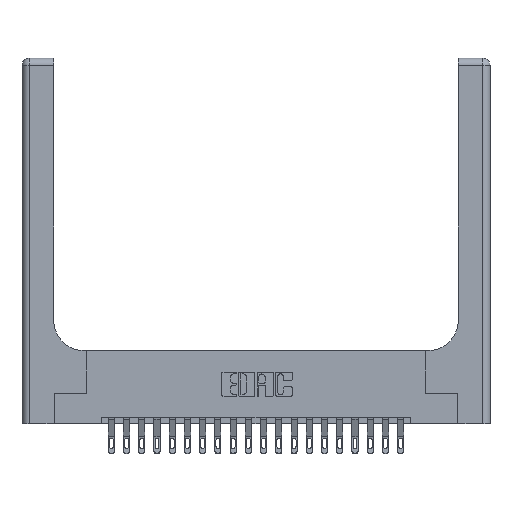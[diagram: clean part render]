
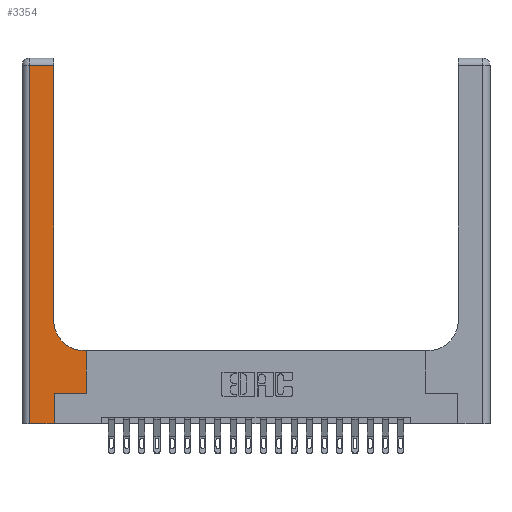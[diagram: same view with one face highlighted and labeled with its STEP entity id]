
A CAD part, top view. The second image highlights one B-rep face of the part: STEP entity #3354.
In plain terms, the highlighted planar face has unit normal (0, 0, 1).
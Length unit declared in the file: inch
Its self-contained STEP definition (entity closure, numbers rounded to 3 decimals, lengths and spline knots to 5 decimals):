
#158 = DIRECTION ( 'NONE',  ( 0., 1., 0. ) ) ;
#617 = DIRECTION ( 'NONE',  ( 0., 1., 0. ) ) ;
#770 = VERTEX_POINT ( 'NONE', #4669 ) ;
#783 = VECTOR ( 'NONE', #617, 39.37008 ) ;
#978 = ORIENTED_EDGE ( 'NONE', *, *, #3199, .T. ) ;
#1184 = CARTESIAN_POINT ( 'NONE',  ( 0.265, 0.25, 0.37 ) ) ;
#1213 = EDGE_CURVE ( 'NONE', #14390, #5880, #8174, .T. ) ;
#1715 = DIRECTION ( 'NONE',  ( 0., 1., 0. ) ) ;
#1854 = VERTEX_POINT ( 'NONE', #5605 ) ;
#2528 = EDGE_CURVE ( 'NONE', #5880, #2581, #20849, .T. ) ;
#2580 = CARTESIAN_POINT ( 'NONE',  ( 0., 0., 0.37 ) ) ;
#2581 = VERTEX_POINT ( 'NONE', #12639 ) ;
#2617 = VECTOR ( 'NONE', #18148, 39.37008 ) ;
#3199 = EDGE_CURVE ( 'NONE', #2581, #13052, #21910, .T. ) ;
#3354 = ADVANCED_FACE ( 'NONE', ( #7127 ), #10811, .F. ) ;
#3676 = VECTOR ( 'NONE', #3851, 39.37008 ) ;
#3730 = LINE ( 'NONE', #15426, #5581 ) ;
#3851 = DIRECTION ( 'NONE',  ( -1., 0., 0. ) ) ;
#4039 = ORIENTED_EDGE ( 'NONE', *, *, #1213, .T. ) ;
#4100 = VECTOR ( 'NONE', #14975, 39.37008 ) ;
#4532 = CARTESIAN_POINT ( 'NONE',  ( 0.51, 0.85, 0.37 ) ) ;
#4669 = CARTESIAN_POINT ( 'NONE',  ( 0.06, 2.94, 0.37 ) ) ;
#5200 = CARTESIAN_POINT ( 'NONE',  ( 0.26, 2.94, 0.37 ) ) ;
#5533 = CARTESIAN_POINT ( 'NONE',  ( 0., 2.94, 0.37 ) ) ;
#5581 = VECTOR ( 'NONE', #158, 39.37008 ) ;
#5605 = CARTESIAN_POINT ( 'NONE',  ( 0.265, 0., 0.37 ) ) ;
#5880 = VERTEX_POINT ( 'NONE', #6760 ) ;
#6688 = VERTEX_POINT ( 'NONE', #11635 ) ;
#6692 = AXIS2_PLACEMENT_3D ( 'NONE', #20903, #9017, #18908 ) ;
#6760 = CARTESIAN_POINT ( 'NONE',  ( 0.528, 0.25, 0.37 ) ) ;
#7127 = FACE_OUTER_BOUND ( 'NONE', #17391, .T. ) ;
#7720 = ORIENTED_EDGE ( 'NONE', *, *, #15344, .T. ) ;
#8174 = LINE ( 'NONE', #18402, #4100 ) ;
#8214 = VERTEX_POINT ( 'NONE', #11285 ) ;
#8620 = VECTOR ( 'NONE', #1715, 39.37008 ) ;
#9017 = DIRECTION ( 'NONE',  ( 0., 0., -1. ) ) ;
#10811 = PLANE ( 'NONE',  #6692 ) ;
#11133 = EDGE_CURVE ( 'NONE', #13052, #8214, #12882, .T. ) ;
#11285 = CARTESIAN_POINT ( 'NONE',  ( 0.26, 0.85, 0.37 ) ) ;
#11506 = CARTESIAN_POINT ( 'NONE',  ( 0.06, 3., 0.37 ) ) ;
#11635 = CARTESIAN_POINT ( 'NONE',  ( 0.06, 0., 0.37 ) ) ;
#11668 = ORIENTED_EDGE ( 'NONE', *, *, #20123, .T. ) ;
#11741 = LINE ( 'NONE', #16849, #8620 ) ;
#12639 = CARTESIAN_POINT ( 'NONE',  ( 0.528, 0.6, 0.37 ) ) ;
#12882 = CIRCLE ( 'NONE', #21733, 0.25 ) ;
#13052 = VERTEX_POINT ( 'NONE', #17190 ) ;
#13332 = ORIENTED_EDGE ( 'NONE', *, *, #13806, .T. ) ;
#13486 = CARTESIAN_POINT ( 'NONE',  ( 0.26, 0.6, 0.37 ) ) ;
#13806 = EDGE_CURVE ( 'NONE', #1854, #14390, #11741, .T. ) ;
#13875 = LINE ( 'NONE', #5533, #3676 ) ;
#14360 = ORIENTED_EDGE ( 'NONE', *, *, #15170, .T. ) ;
#14390 = VERTEX_POINT ( 'NONE', #1184 ) ;
#14546 = EDGE_CURVE ( 'NONE', #21934, #770, #13875, .T. ) ;
#14562 = DIRECTION ( 'NONE',  ( 0., 0., -1. ) ) ;
#14975 = DIRECTION ( 'NONE',  ( 1., 0., 0. ) ) ;
#15170 = EDGE_CURVE ( 'NONE', #6688, #1854, #19482, .T. ) ;
#15344 = EDGE_CURVE ( 'NONE', #770, #6688, #18474, .T. ) ;
#15426 = CARTESIAN_POINT ( 'NONE',  ( 0.26, 3., 0.37 ) ) ;
#15474 = ORIENTED_EDGE ( 'NONE', *, *, #14546, .T. ) ;
#15646 = CARTESIAN_POINT ( 'NONE',  ( 0.528, 0.25, 0.37 ) ) ;
#16166 = DIRECTION ( 'NONE',  ( 1., 0., 0. ) ) ;
#16849 = CARTESIAN_POINT ( 'NONE',  ( 0.265, 0., 0.37 ) ) ;
#16992 = ORIENTED_EDGE ( 'NONE', *, *, #11133, .T. ) ;
#17190 = CARTESIAN_POINT ( 'NONE',  ( 0.51, 0.6, 0.37 ) ) ;
#17391 = EDGE_LOOP ( 'NONE', ( #11668, #15474, #7720, #14360, #13332, #4039, #17827, #978, #16992 ) ) ;
#17827 = ORIENTED_EDGE ( 'NONE', *, *, #2528, .T. ) ;
#18148 = DIRECTION ( 'NONE',  ( 0., -1., 0. ) ) ;
#18402 = CARTESIAN_POINT ( 'NONE',  ( 0.265, 0.25, 0.37 ) ) ;
#18474 = LINE ( 'NONE', #11506, #2617 ) ;
#18908 = DIRECTION ( 'NONE',  ( -1., 0., 0. ) ) ;
#19327 = VECTOR ( 'NONE', #16166, 39.37008 ) ;
#19331 = DIRECTION ( 'NONE',  ( 1., 0., 0. ) ) ;
#19482 = LINE ( 'NONE', #2580, #19327 ) ;
#20123 = EDGE_CURVE ( 'NONE', #8214, #21934, #3730, .T. ) ;
#20246 = DIRECTION ( 'NONE',  ( -1., 0., 0. ) ) ;
#20849 = LINE ( 'NONE', #15646, #783 ) ;
#20903 = CARTESIAN_POINT ( 'NONE',  ( 0., 3., 0.37 ) ) ;
#21505 = VECTOR ( 'NONE', #20246, 39.37008 ) ;
#21733 = AXIS2_PLACEMENT_3D ( 'NONE', #4532, #14562, #19331 ) ;
#21910 = LINE ( 'NONE', #13486, #21505 ) ;
#21934 = VERTEX_POINT ( 'NONE', #5200 ) ;
